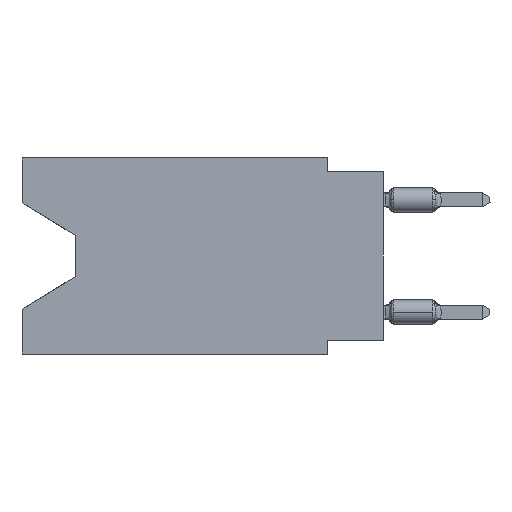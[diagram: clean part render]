
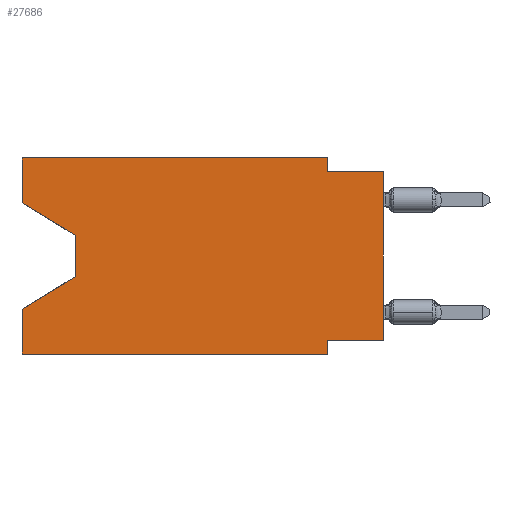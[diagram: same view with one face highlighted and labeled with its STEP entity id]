
A CAD part, left-side view. The second image highlights one B-rep face of the part: STEP entity #27686.
In plain terms, the highlighted planar face has unit normal (-1, 0, 0).
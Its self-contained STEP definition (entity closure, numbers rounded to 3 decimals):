
#502 = VECTOR ( 'NONE', #26145, 1000. ) ;
#537 = CARTESIAN_POINT ( 'NONE',  ( 0., 16.383, -2.038 ) ) ;
#723 = VERTEX_POINT ( 'NONE', #7856 ) ;
#923 = LINE ( 'NONE', #3417, #7219 ) ;
#969 = CARTESIAN_POINT ( 'NONE',  ( 0., 2.54, 0. ) ) ;
#1952 = EDGE_LOOP ( 'NONE', ( #30963, #12673, #29984, #11713, #10658, #32865, #23426, #24203, #29453, #11973, #26922, #24113 ) ) ;
#2222 = VERTEX_POINT ( 'NONE', #969 ) ;
#2906 = CARTESIAN_POINT ( 'NONE',  ( 0., 2.54, -8.89 ) ) ;
#3195 = CARTESIAN_POINT ( 'NONE',  ( 0., 13.97, -3.505 ) ) ;
#3239 = DIRECTION ( 'NONE',  ( 0., 0., 1. ) ) ;
#3417 = CARTESIAN_POINT ( 'NONE',  ( 0., 16.383, 0. ) ) ;
#3572 = CARTESIAN_POINT ( 'NONE',  ( 0., 16.383, -8.89 ) ) ;
#3688 = DIRECTION ( 'NONE',  ( 0., 0., -1. ) ) ;
#4111 = VERTEX_POINT ( 'NONE', #31904 ) ;
#4139 = EDGE_CURVE ( 'NONE', #16822, #32627, #24753, .T. ) ;
#4267 = CARTESIAN_POINT ( 'NONE',  ( 0., 16.383, -8.89 ) ) ;
#4578 = LINE ( 'NONE', #11436, #30031 ) ;
#5290 = EDGE_CURVE ( 'NONE', #10484, #21239, #11105, .T. ) ;
#5368 = DIRECTION ( 'NONE',  ( 0., 0., -1. ) ) ;
#5505 = VECTOR ( 'NONE', #14449, 1000. ) ;
#5557 = EDGE_CURVE ( 'NONE', #723, #10444, #22756, .T. ) ;
#7219 = VECTOR ( 'NONE', #18270, 1000. ) ;
#7635 = VECTOR ( 'NONE', #21259, 1000. ) ;
#7856 = CARTESIAN_POINT ( 'NONE',  ( 0., 0., -8.255 ) ) ;
#10145 = EDGE_CURVE ( 'NONE', #4111, #2222, #30837, .T. ) ;
#10303 = EDGE_CURVE ( 'NONE', #2222, #17299, #26019, .T. ) ;
#10348 = EDGE_CURVE ( 'NONE', #17117, #29901, #19202, .T. ) ;
#10430 = CARTESIAN_POINT ( 'NONE',  ( 0., 0., 0. ) ) ;
#10444 = VERTEX_POINT ( 'NONE', #19369 ) ;
#10484 = VERTEX_POINT ( 'NONE', #10518 ) ;
#10518 = CARTESIAN_POINT ( 'NONE',  ( 0., 13.97, -5.385 ) ) ;
#10658 = ORIENTED_EDGE ( 'NONE', *, *, #4139, .T. ) ;
#10816 = CARTESIAN_POINT ( 'NONE',  ( 0., 16.383, 0. ) ) ;
#11105 = LINE ( 'NONE', #26252, #7635 ) ;
#11152 = VECTOR ( 'NONE', #3239, 1000. ) ;
#11164 = EDGE_CURVE ( 'NONE', #17117, #4111, #18428, .T. ) ;
#11367 = EDGE_CURVE ( 'NONE', #723, #11584, #17578, .T. ) ;
#11436 = CARTESIAN_POINT ( 'NONE',  ( 0., 0., -0.635 ) ) ;
#11584 = VERTEX_POINT ( 'NONE', #26823 ) ;
#11713 = ORIENTED_EDGE ( 'NONE', *, *, #25235, .F. ) ;
#11973 = ORIENTED_EDGE ( 'NONE', *, *, #10303, .F. ) ;
#12182 = AXIS2_PLACEMENT_3D ( 'NONE', #10816, #30942, #25810 ) ;
#12673 = ORIENTED_EDGE ( 'NONE', *, *, #16574, .T. ) ;
#13435 = LINE ( 'NONE', #18113, #30083 ) ;
#14449 = DIRECTION ( 'NONE',  ( 0., -1., 0. ) ) ;
#14950 = CARTESIAN_POINT ( 'NONE',  ( 0., 16.383, 0. ) ) ;
#16551 = CARTESIAN_POINT ( 'NONE',  ( 0., 2.54, 0. ) ) ;
#16574 = EDGE_CURVE ( 'NONE', #29901, #10484, #31165, .T. ) ;
#16822 = VERTEX_POINT ( 'NONE', #3572 ) ;
#16887 = CARTESIAN_POINT ( 'NONE',  ( 0., 16.383, -2.038 ) ) ;
#16906 = VECTOR ( 'NONE', #3688, 1000. ) ;
#17117 = VERTEX_POINT ( 'NONE', #537 ) ;
#17299 = VERTEX_POINT ( 'NONE', #28837 ) ;
#17578 = LINE ( 'NONE', #20070, #502 ) ;
#18006 = FACE_OUTER_BOUND ( 'NONE', #1952, .T. ) ;
#18113 = CARTESIAN_POINT ( 'NONE',  ( 0., 2.54, -8.89 ) ) ;
#18270 = DIRECTION ( 'NONE',  ( 0., 0., 1. ) ) ;
#18428 = LINE ( 'NONE', #21236, #11152 ) ;
#18960 = VECTOR ( 'NONE', #5368, 1000. ) ;
#19202 = LINE ( 'NONE', #16887, #26983 ) ;
#19369 = CARTESIAN_POINT ( 'NONE',  ( 0., 0., -0.635 ) ) ;
#19432 = DIRECTION ( 'NONE',  ( 0., -1., 0. ) ) ;
#19789 = EDGE_CURVE ( 'NONE', #17299, #10444, #4578, .T. ) ;
#20070 = CARTESIAN_POINT ( 'NONE',  ( 0., 0., -8.255 ) ) ;
#20251 = DIRECTION ( 'NONE',  ( 0., 0., 1. ) ) ;
#20651 = PLANE ( 'NONE',  #12182 ) ;
#20715 = CARTESIAN_POINT ( 'NONE',  ( 0., 16.383, -6.852 ) ) ;
#21114 = VECTOR ( 'NONE', #32400, 1000. ) ;
#21236 = CARTESIAN_POINT ( 'NONE',  ( 0., 16.383, 0. ) ) ;
#21239 = VERTEX_POINT ( 'NONE', #20715 ) ;
#21259 = DIRECTION ( 'NONE',  ( 0., 0.855, -0.519 ) ) ;
#22756 = LINE ( 'NONE', #10430, #30511 ) ;
#23426 = ORIENTED_EDGE ( 'NONE', *, *, #11367, .F. ) ;
#23840 = CARTESIAN_POINT ( 'NONE',  ( 0., 13.97, -3.505 ) ) ;
#24113 = ORIENTED_EDGE ( 'NONE', *, *, #11164, .F. ) ;
#24203 = ORIENTED_EDGE ( 'NONE', *, *, #5557, .T. ) ;
#24753 = LINE ( 'NONE', #4267, #5505 ) ;
#25235 = EDGE_CURVE ( 'NONE', #16822, #21239, #923, .T. ) ;
#25300 = EDGE_CURVE ( 'NONE', #11584, #32627, #13435, .T. ) ;
#25810 = DIRECTION ( 'NONE',  ( 0., 0., -1. ) ) ;
#26019 = LINE ( 'NONE', #16551, #16906 ) ;
#26145 = DIRECTION ( 'NONE',  ( 0., 1., 0. ) ) ;
#26252 = CARTESIAN_POINT ( 'NONE',  ( 0., 13.97, -5.385 ) ) ;
#26823 = CARTESIAN_POINT ( 'NONE',  ( 0., 2.54, -8.255 ) ) ;
#26922 = ORIENTED_EDGE ( 'NONE', *, *, #10145, .F. ) ;
#26983 = VECTOR ( 'NONE', #32321, 1000. ) ;
#27686 = ADVANCED_FACE ( 'NONE', ( #18006 ), #20651, .F. ) ;
#28837 = CARTESIAN_POINT ( 'NONE',  ( 0., 2.54, -0.635 ) ) ;
#29453 = ORIENTED_EDGE ( 'NONE', *, *, #19789, .F. ) ;
#29901 = VERTEX_POINT ( 'NONE', #23840 ) ;
#29984 = ORIENTED_EDGE ( 'NONE', *, *, #5290, .T. ) ;
#30031 = VECTOR ( 'NONE', #19432, 1000. ) ;
#30083 = VECTOR ( 'NONE', #30895, 1000. ) ;
#30511 = VECTOR ( 'NONE', #20251, 1000. ) ;
#30837 = LINE ( 'NONE', #14950, #21114 ) ;
#30895 = DIRECTION ( 'NONE',  ( 0., 0., -1. ) ) ;
#30942 = DIRECTION ( 'NONE',  ( 1., 0., 0. ) ) ;
#30963 = ORIENTED_EDGE ( 'NONE', *, *, #10348, .T. ) ;
#31165 = LINE ( 'NONE', #3195, #18960 ) ;
#31904 = CARTESIAN_POINT ( 'NONE',  ( 0., 16.383, 0. ) ) ;
#32321 = DIRECTION ( 'NONE',  ( 0., -0.855, -0.519 ) ) ;
#32400 = DIRECTION ( 'NONE',  ( 0., -1., 0. ) ) ;
#32627 = VERTEX_POINT ( 'NONE', #2906 ) ;
#32865 = ORIENTED_EDGE ( 'NONE', *, *, #25300, .F. ) ;
